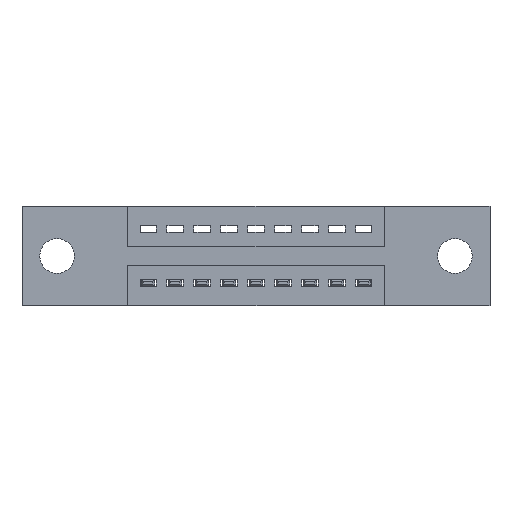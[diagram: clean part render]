
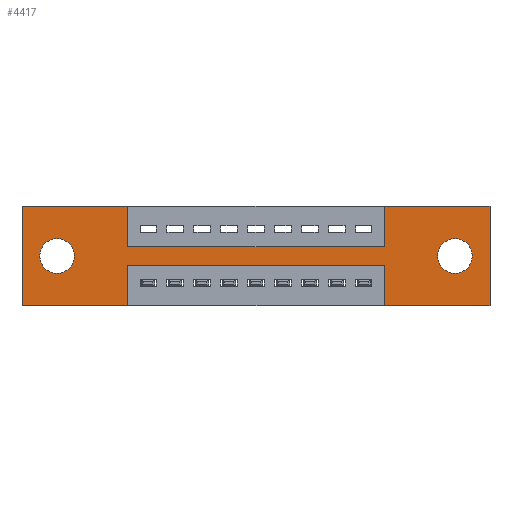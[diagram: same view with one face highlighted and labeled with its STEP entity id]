
A CAD part, front view. The second image highlights one B-rep face of the part: STEP entity #4417.
In plain terms, the highlighted planar face has unit normal (0, -1, 0).
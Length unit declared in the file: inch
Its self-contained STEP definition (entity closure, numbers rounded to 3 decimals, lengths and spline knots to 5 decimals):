
#6 = AXIS2_PLACEMENT_3D ( 'NONE', #3216, #1660, #4081 ) ;
#27 = CARTESIAN_POINT ( 'NONE',  ( 0., 0., 0. ) ) ;
#66 = ORIENTED_EDGE ( 'NONE', *, *, #8711, .F. ) ;
#116 = CIRCLE ( 'NONE', #6, 0.064 ) ;
#158 = LINE ( 'NONE', #4629, #8943 ) ;
#245 = CIRCLE ( 'NONE', #1629, 0.064 ) ;
#497 = LINE ( 'NONE', #1022, #10910 ) ;
#507 = FACE_BOUND ( 'NONE', #7379, .T. ) ;
#611 = VERTEX_POINT ( 'NONE', #9665 ) ;
#901 = VERTEX_POINT ( 'NONE', #8714 ) ;
#947 = CARTESIAN_POINT ( 'NONE',  ( 1.735, 0., -0.37 ) ) ;
#1022 = CARTESIAN_POINT ( 'NONE',  ( 1.3425, 0., -0.37 ) ) ;
#1027 = DIRECTION ( 'NONE',  ( -1., 0., 0. ) ) ;
#1181 = ORIENTED_EDGE ( 'NONE', *, *, #5332, .F. ) ;
#1356 = CARTESIAN_POINT ( 'NONE',  ( 0.13, 0., -0.185 ) ) ;
#1380 = CARTESIAN_POINT ( 'NONE',  ( 0., 0., 0. ) ) ;
#1426 = LINE ( 'NONE', #4116, #11036 ) ;
#1605 = VECTOR ( 'NONE', #1027, 39.37008 ) ;
#1624 = CARTESIAN_POINT ( 'NONE',  ( 1.605, 0., -0.249 ) ) ;
#1629 = AXIS2_PLACEMENT_3D ( 'NONE', #1356, #8290, #6449 ) ;
#1655 = ORIENTED_EDGE ( 'NONE', *, *, #10146, .T. ) ;
#1660 = DIRECTION ( 'NONE',  ( 0., 1., 0. ) ) ;
#1861 = DIRECTION ( 'NONE',  ( 0., 0., 1. ) ) ;
#1887 = DIRECTION ( 'NONE',  ( 1., 0., 0. ) ) ;
#1956 = VERTEX_POINT ( 'NONE', #8484 ) ;
#2079 = CARTESIAN_POINT ( 'NONE',  ( 0.3925, 0., -0.22 ) ) ;
#2151 = EDGE_CURVE ( 'NONE', #9655, #5213, #6793, .T. ) ;
#2361 = VECTOR ( 'NONE', #11052, 39.37008 ) ;
#2570 = EDGE_CURVE ( 'NONE', #6920, #4800, #3436, .T. ) ;
#2623 = CARTESIAN_POINT ( 'NONE',  ( 0.3925, 0., -0.15 ) ) ;
#2698 = EDGE_CURVE ( 'NONE', #3397, #901, #9926, .T. ) ;
#2760 = CARTESIAN_POINT ( 'NONE',  ( 0., 0., 0. ) ) ;
#2785 = AXIS2_PLACEMENT_3D ( 'NONE', #8222, #3876, #6494 ) ;
#2836 = CARTESIAN_POINT ( 'NONE',  ( 0.3925, 0., -0.22 ) ) ;
#2932 = CARTESIAN_POINT ( 'NONE',  ( 0.3925, 0., -0.37 ) ) ;
#2956 = CARTESIAN_POINT ( 'NONE',  ( 0., 0., -0.37 ) ) ;
#3050 = VECTOR ( 'NONE', #10808, 39.37008 ) ;
#3071 = DIRECTION ( 'NONE',  ( 0., 0., 1. ) ) ;
#3216 = CARTESIAN_POINT ( 'NONE',  ( 0.13, 0., -0.185 ) ) ;
#3224 = CARTESIAN_POINT ( 'NONE',  ( 0.13, 0., -0.121 ) ) ;
#3305 = VECTOR ( 'NONE', #6299, 39.37008 ) ;
#3349 = EDGE_CURVE ( 'NONE', #901, #10404, #10418, .T. ) ;
#3397 = VERTEX_POINT ( 'NONE', #27 ) ;
#3436 = LINE ( 'NONE', #2760, #10042 ) ;
#3462 = PLANE ( 'NONE',  #10879 ) ;
#3519 = CARTESIAN_POINT ( 'NONE',  ( 1.3425, 0., -0.15 ) ) ;
#3541 = LINE ( 'NONE', #9552, #8899 ) ;
#3553 = CIRCLE ( 'NONE', #2785, 0.064 ) ;
#3876 = DIRECTION ( 'NONE',  ( 0., 1., 0. ) ) ;
#3944 = AXIS2_PLACEMENT_3D ( 'NONE', #9400, #7669, #6749 ) ;
#4006 = ORIENTED_EDGE ( 'NONE', *, *, #4286, .F. ) ;
#4057 = EDGE_CURVE ( 'NONE', #5365, #5695, #116, .T. ) ;
#4081 = DIRECTION ( 'NONE',  ( 0., 0., 1. ) ) ;
#4099 = VERTEX_POINT ( 'NONE', #1624 ) ;
#4116 = CARTESIAN_POINT ( 'NONE',  ( 0., 0., -0.37 ) ) ;
#4286 = EDGE_CURVE ( 'NONE', #611, #3397, #10658, .T. ) ;
#4318 = CARTESIAN_POINT ( 'NONE',  ( 0.3925, 0., 0. ) ) ;
#4398 = EDGE_LOOP ( 'NONE', ( #1655, #10697 ) ) ;
#4417 = ADVANCED_FACE ( 'NONE', ( #4757, #507, #7662 ), #3462, .T. ) ;
#4423 = CARTESIAN_POINT ( 'NONE',  ( 1.605, 0., -0.121 ) ) ;
#4433 = CARTESIAN_POINT ( 'NONE',  ( 0., 0., -0.37 ) ) ;
#4539 = CARTESIAN_POINT ( 'NONE',  ( 1.3425, 0., -0.37 ) ) ;
#4629 = CARTESIAN_POINT ( 'NONE',  ( 0.3925, 0., -0.15 ) ) ;
#4664 = ORIENTED_EDGE ( 'NONE', *, *, #9404, .F. ) ;
#4757 = FACE_BOUND ( 'NONE', #4398, .T. ) ;
#4800 = VERTEX_POINT ( 'NONE', #10377 ) ;
#5136 = ORIENTED_EDGE ( 'NONE', *, *, #8638, .F. ) ;
#5207 = EDGE_CURVE ( 'NONE', #5695, #5365, #245, .T. ) ;
#5213 = VERTEX_POINT ( 'NONE', #2079 ) ;
#5222 = EDGE_CURVE ( 'NONE', #1956, #611, #1426, .T. ) ;
#5306 = ORIENTED_EDGE ( 'NONE', *, *, #2698, .F. ) ;
#5332 = EDGE_CURVE ( 'NONE', #7657, #9655, #497, .T. ) ;
#5365 = VERTEX_POINT ( 'NONE', #8755 ) ;
#5500 = DIRECTION ( 'NONE',  ( 1., 0., 0. ) ) ;
#5695 = VERTEX_POINT ( 'NONE', #3224 ) ;
#5719 = DIRECTION ( 'NONE',  ( 0., 0., 1. ) ) ;
#5927 = ORIENTED_EDGE ( 'NONE', *, *, #5222, .F. ) ;
#6299 = DIRECTION ( 'NONE',  ( -1., 0., 0. ) ) ;
#6378 = VECTOR ( 'NONE', #5719, 39.37008 ) ;
#6449 = DIRECTION ( 'NONE',  ( 0., 0., 1. ) ) ;
#6494 = DIRECTION ( 'NONE',  ( 0., 0., -1. ) ) ;
#6530 = VERTEX_POINT ( 'NONE', #947 ) ;
#6749 = DIRECTION ( 'NONE',  ( 0., 0., -1. ) ) ;
#6793 = LINE ( 'NONE', #2836, #1605 ) ;
#6915 = ORIENTED_EDGE ( 'NONE', *, *, #5207, .T. ) ;
#6920 = VERTEX_POINT ( 'NONE', #8360 ) ;
#7012 = LINE ( 'NONE', #10136, #6378 ) ;
#7046 = ORIENTED_EDGE ( 'NONE', *, *, #10718, .F. ) ;
#7135 = DIRECTION ( 'NONE',  ( 0., 0., -1. ) ) ;
#7379 = EDGE_LOOP ( 'NONE', ( #6915, #9011 ) ) ;
#7657 = VERTEX_POINT ( 'NONE', #4539 ) ;
#7662 = FACE_OUTER_BOUND ( 'NONE', #7885, .T. ) ;
#7669 = DIRECTION ( 'NONE',  ( 0., 1., 0. ) ) ;
#7885 = EDGE_LOOP ( 'NONE', ( #66, #9417, #1181, #4664, #8830, #9984, #7046, #5136, #8993, #5306, #4006, #5927 ) ) ;
#7958 = CIRCLE ( 'NONE', #3944, 0.064 ) ;
#8142 = CARTESIAN_POINT ( 'NONE',  ( 0., 0., 0. ) ) ;
#8222 = CARTESIAN_POINT ( 'NONE',  ( 1.605, 0., -0.185 ) ) ;
#8290 = DIRECTION ( 'NONE',  ( 0., 1., 0. ) ) ;
#8360 = CARTESIAN_POINT ( 'NONE',  ( 1.3425, 0., 0. ) ) ;
#8379 = DIRECTION ( 'NONE',  ( -1., 0., 0. ) ) ;
#8382 = LINE ( 'NONE', #2932, #10047 ) ;
#8484 = CARTESIAN_POINT ( 'NONE',  ( 0.3925, 0., -0.37 ) ) ;
#8638 = EDGE_CURVE ( 'NONE', #10404, #10922, #158, .T. ) ;
#8711 = EDGE_CURVE ( 'NONE', #5213, #1956, #8382, .T. ) ;
#8714 = CARTESIAN_POINT ( 'NONE',  ( 0.3925, 0., 0. ) ) ;
#8755 = CARTESIAN_POINT ( 'NONE',  ( 0.13, 0., -0.249 ) ) ;
#8830 = ORIENTED_EDGE ( 'NONE', *, *, #10968, .F. ) ;
#8899 = VECTOR ( 'NONE', #10432, 39.37008 ) ;
#8922 = LINE ( 'NONE', #2956, #3305 ) ;
#8943 = VECTOR ( 'NONE', #5500, 39.37008 ) ;
#8993 = ORIENTED_EDGE ( 'NONE', *, *, #3349, .F. ) ;
#9011 = ORIENTED_EDGE ( 'NONE', *, *, #4057, .T. ) ;
#9241 = DIRECTION ( 'NONE',  ( 0., 0., -1. ) ) ;
#9400 = CARTESIAN_POINT ( 'NONE',  ( 1.605, 0., -0.185 ) ) ;
#9404 = EDGE_CURVE ( 'NONE', #6530, #7657, #8922, .T. ) ;
#9417 = ORIENTED_EDGE ( 'NONE', *, *, #2151, .F. ) ;
#9552 = CARTESIAN_POINT ( 'NONE',  ( 1.735, 0., 0. ) ) ;
#9655 = VERTEX_POINT ( 'NONE', #10380 ) ;
#9665 = CARTESIAN_POINT ( 'NONE',  ( 0., 0., -0.37 ) ) ;
#9926 = LINE ( 'NONE', #8142, #3050 ) ;
#9984 = ORIENTED_EDGE ( 'NONE', *, *, #2570, .F. ) ;
#10007 = VECTOR ( 'NONE', #3071, 39.37008 ) ;
#10042 = VECTOR ( 'NONE', #1887, 39.37008 ) ;
#10047 = VECTOR ( 'NONE', #7135, 39.37008 ) ;
#10136 = CARTESIAN_POINT ( 'NONE',  ( 1.3425, 0., 0. ) ) ;
#10146 = EDGE_CURVE ( 'NONE', #10360, #4099, #7958, .T. ) ;
#10335 = DIRECTION ( 'NONE',  ( 0., -1., 0. ) ) ;
#10360 = VERTEX_POINT ( 'NONE', #4423 ) ;
#10377 = CARTESIAN_POINT ( 'NONE',  ( 1.735, 0., 0. ) ) ;
#10380 = CARTESIAN_POINT ( 'NONE',  ( 1.3425, 0., -0.22 ) ) ;
#10404 = VERTEX_POINT ( 'NONE', #2623 ) ;
#10418 = LINE ( 'NONE', #4318, #2361 ) ;
#10432 = DIRECTION ( 'NONE',  ( 0., 0., -1. ) ) ;
#10567 = EDGE_CURVE ( 'NONE', #4099, #10360, #3553, .T. ) ;
#10658 = LINE ( 'NONE', #1380, #10007 ) ;
#10697 = ORIENTED_EDGE ( 'NONE', *, *, #10567, .T. ) ;
#10718 = EDGE_CURVE ( 'NONE', #10922, #6920, #7012, .T. ) ;
#10808 = DIRECTION ( 'NONE',  ( 1., 0., 0. ) ) ;
#10879 = AXIS2_PLACEMENT_3D ( 'NONE', #4433, #10335, #9241 ) ;
#10910 = VECTOR ( 'NONE', #1861, 39.37008 ) ;
#10922 = VERTEX_POINT ( 'NONE', #3519 ) ;
#10968 = EDGE_CURVE ( 'NONE', #4800, #6530, #3541, .T. ) ;
#11036 = VECTOR ( 'NONE', #8379, 39.37008 ) ;
#11052 = DIRECTION ( 'NONE',  ( 0., 0., -1. ) ) ;
